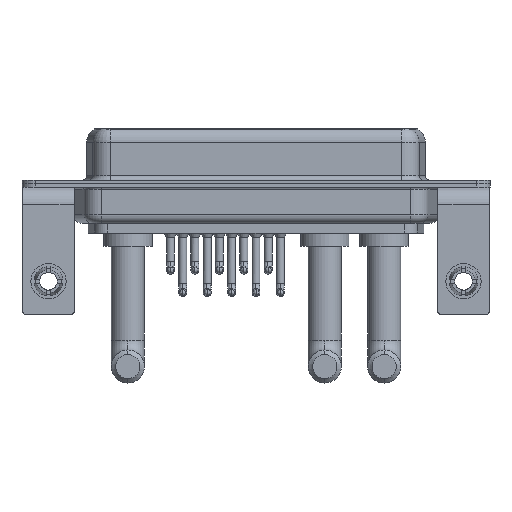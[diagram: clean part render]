
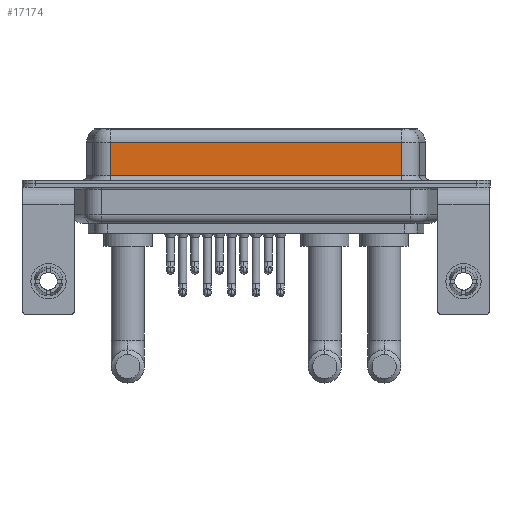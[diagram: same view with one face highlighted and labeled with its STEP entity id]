
A CAD part, front view. The second image highlights one B-rep face of the part: STEP entity #17174.
In plain terms, the highlighted planar face has unit normal (0, -1, 0).
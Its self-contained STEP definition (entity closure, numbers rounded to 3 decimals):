
#2180 = DIRECTION ( 'NONE',  ( 0., 0., -1. ) ) ;
#2570 = LINE ( 'NONE', #4422, #4773 ) ;
#4422 = CARTESIAN_POINT ( 'NONE',  ( 40.037, -3.95, 0.9 ) ) ;
#4728 = DIRECTION ( 'NONE',  ( 0., 0., 1. ) ) ;
#4772 = ORIENTED_EDGE ( 'NONE', *, *, #19305, .F. ) ;
#4773 = VECTOR ( 'NONE', #17752, 1000. ) ;
#5805 = LINE ( 'NONE', #12436, #8118 ) ;
#7461 = VERTEX_POINT ( 'NONE', #17617 ) ;
#7963 = CARTESIAN_POINT ( 'NONE',  ( 7.013, -3.95, 0.9 ) ) ;
#8118 = VECTOR ( 'NONE', #8743, 1000. ) ;
#8408 = CARTESIAN_POINT ( 'NONE',  ( 40.037, -3.95, 4.65 ) ) ;
#8542 = CARTESIAN_POINT ( 'NONE',  ( 7.013, -3.95, 4.65 ) ) ;
#8743 = DIRECTION ( 'NONE',  ( 0., 0., -1. ) ) ;
#9637 = DIRECTION ( 'NONE',  ( -1., 0., 0. ) ) ;
#9743 = LINE ( 'NONE', #8408, #15712 ) ;
#10133 = CARTESIAN_POINT ( 'NONE',  ( 40.037, -3.95, 6.4 ) ) ;
#10470 = CARTESIAN_POINT ( 'NONE',  ( 40.037, -3.95, 0.9 ) ) ;
#11470 = PLANE ( 'NONE',  #14483 ) ;
#11784 = EDGE_CURVE ( 'NONE', #12491, #13103, #5805, .T. ) ;
#12436 = CARTESIAN_POINT ( 'NONE',  ( 7.013, -3.95, 6.4 ) ) ;
#12491 = VERTEX_POINT ( 'NONE', #8542 ) ;
#12663 = ORIENTED_EDGE ( 'NONE', *, *, #16553, .T. ) ;
#13092 = CARTESIAN_POINT ( 'NONE',  ( 40.037, -3.95, 6.4 ) ) ;
#13103 = VERTEX_POINT ( 'NONE', #7963 ) ;
#14483 = AXIS2_PLACEMENT_3D ( 'NONE', #13092, #19877, #4728 ) ;
#14535 = VERTEX_POINT ( 'NONE', #10470 ) ;
#14595 = FACE_OUTER_BOUND ( 'NONE', #17088, .T. ) ;
#15712 = VECTOR ( 'NONE', #9637, 1000. ) ;
#15921 = ORIENTED_EDGE ( 'NONE', *, *, #11784, .T. ) ;
#16553 = EDGE_CURVE ( 'NONE', #13103, #14535, #2570, .T. ) ;
#16912 = ORIENTED_EDGE ( 'NONE', *, *, #19975, .T. ) ;
#17023 = LINE ( 'NONE', #10133, #20855 ) ;
#17088 = EDGE_LOOP ( 'NONE', ( #4772, #16912, #15921, #12663 ) ) ;
#17174 = ADVANCED_FACE ( 'NONE', ( #14595 ), #11470, .F. ) ;
#17617 = CARTESIAN_POINT ( 'NONE',  ( 40.037, -3.95, 4.65 ) ) ;
#17752 = DIRECTION ( 'NONE',  ( 1., 0., 0. ) ) ;
#19305 = EDGE_CURVE ( 'NONE', #7461, #14535, #17023, .T. ) ;
#19877 = DIRECTION ( 'NONE',  ( 0., 1., 0. ) ) ;
#19975 = EDGE_CURVE ( 'NONE', #7461, #12491, #9743, .T. ) ;
#20855 = VECTOR ( 'NONE', #2180, 1000. ) ;
